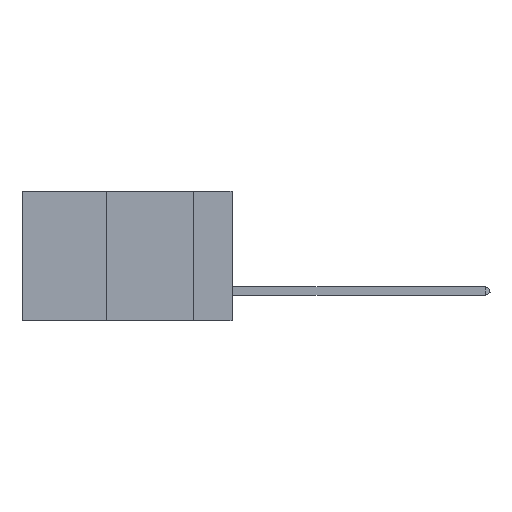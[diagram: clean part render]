
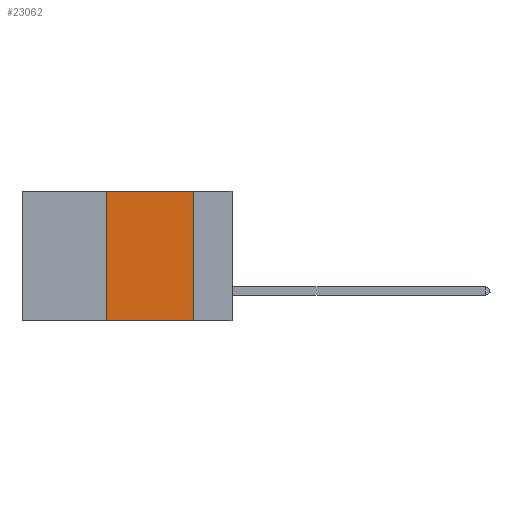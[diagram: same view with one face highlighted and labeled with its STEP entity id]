
A CAD part, left-side view. The second image highlights one B-rep face of the part: STEP entity #23062.
In plain terms, the highlighted planar face has unit normal (-1, 0, 0).
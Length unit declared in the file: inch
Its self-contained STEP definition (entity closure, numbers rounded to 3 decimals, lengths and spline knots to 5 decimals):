
#574 = CARTESIAN_POINT ( 'NONE',  ( 0., 0.6, -0.37 ) ) ;
#1947 = CARTESIAN_POINT ( 'NONE',  ( 0., 0.11, 0. ) ) ;
#2976 = CARTESIAN_POINT ( 'NONE',  ( 0., 0.36, 0. ) ) ;
#3536 = ORIENTED_EDGE ( 'NONE', *, *, #15549, .F. ) ;
#5032 = CARTESIAN_POINT ( 'NONE',  ( 0., 0.11, 0. ) ) ;
#5404 = ORIENTED_EDGE ( 'NONE', *, *, #8616, .F. ) ;
#6620 = DIRECTION ( 'NONE',  ( 0., 0., 1. ) ) ;
#6750 = AXIS2_PLACEMENT_3D ( 'NONE', #15822, #12487, #14289 ) ;
#6936 = DIRECTION ( 'NONE',  ( 0., -1., 0. ) ) ;
#7200 = VERTEX_POINT ( 'NONE', #14626 ) ;
#7220 = LINE ( 'NONE', #2976, #8312 ) ;
#7950 = ORIENTED_EDGE ( 'NONE', *, *, #18810, .T. ) ;
#8312 = VECTOR ( 'NONE', #6620, 39.37008 ) ;
#8440 = ORIENTED_EDGE ( 'NONE', *, *, #15523, .F. ) ;
#8616 = EDGE_CURVE ( 'NONE', #18022, #19803, #10454, .T. ) ;
#9262 = VERTEX_POINT ( 'NONE', #11573 ) ;
#9741 = LINE ( 'NONE', #574, #22235 ) ;
#10454 = LINE ( 'NONE', #19535, #15471 ) ;
#11573 = CARTESIAN_POINT ( 'NONE',  ( 0., 0.36, -0.37 ) ) ;
#11791 = CARTESIAN_POINT ( 'NONE',  ( 0., 0.36, 0. ) ) ;
#11862 = FACE_OUTER_BOUND ( 'NONE', #12889, .T. ) ;
#12487 = DIRECTION ( 'NONE',  ( 1., 0., 0. ) ) ;
#12889 = EDGE_LOOP ( 'NONE', ( #8440, #5404, #3536, #7950 ) ) ;
#14289 = DIRECTION ( 'NONE',  ( 0., 0., -1. ) ) ;
#14367 = PLANE ( 'NONE',  #6750 ) ;
#14626 = CARTESIAN_POINT ( 'NONE',  ( 0., 0.11, -0.37 ) ) ;
#15471 = VECTOR ( 'NONE', #6936, 39.37008 ) ;
#15523 = EDGE_CURVE ( 'NONE', #19803, #7200, #17777, .T. ) ;
#15539 = DIRECTION ( 'NONE',  ( 0., 0., -1. ) ) ;
#15549 = EDGE_CURVE ( 'NONE', #9262, #18022, #7220, .T. ) ;
#15822 = CARTESIAN_POINT ( 'NONE',  ( 0., 0.6, 0. ) ) ;
#16364 = DIRECTION ( 'NONE',  ( 0., -1., 0. ) ) ;
#17226 = VECTOR ( 'NONE', #15539, 39.37008 ) ;
#17777 = LINE ( 'NONE', #5032, #17226 ) ;
#18022 = VERTEX_POINT ( 'NONE', #11791 ) ;
#18810 = EDGE_CURVE ( 'NONE', #9262, #7200, #9741, .T. ) ;
#19535 = CARTESIAN_POINT ( 'NONE',  ( 0., 0.6, 0. ) ) ;
#19803 = VERTEX_POINT ( 'NONE', #1947 ) ;
#22235 = VECTOR ( 'NONE', #16364, 39.37008 ) ;
#23062 = ADVANCED_FACE ( 'NONE', ( #11862 ), #14367, .F. ) ;
